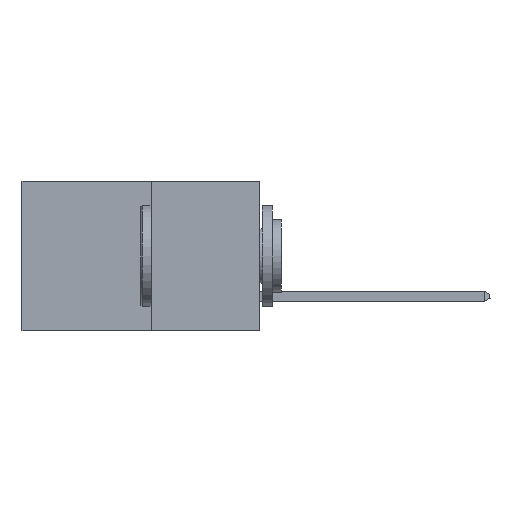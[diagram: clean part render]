
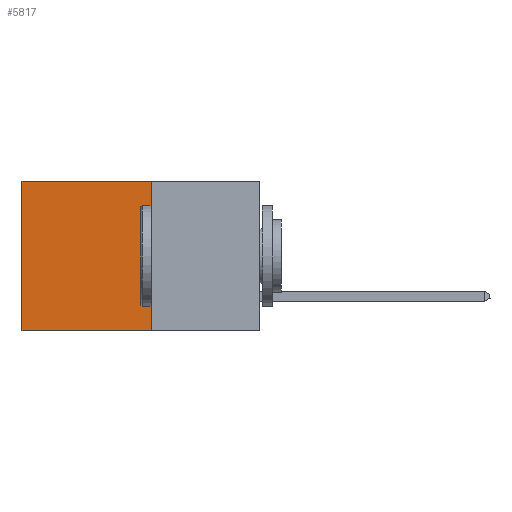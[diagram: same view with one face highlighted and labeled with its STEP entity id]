
A CAD part, left-side view. The second image highlights one B-rep face of the part: STEP entity #5817.
In plain terms, the highlighted planar face has unit normal (-1, 0, 0).
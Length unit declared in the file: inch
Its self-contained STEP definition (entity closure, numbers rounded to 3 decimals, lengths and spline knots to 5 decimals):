
#403 = EDGE_CURVE ( 'NONE', #16762, #11495, #9783, .T. ) ;
#775 = LINE ( 'NONE', #1571, #11149 ) ;
#1303 = FACE_OUTER_BOUND ( 'NONE', #5108, .T. ) ;
#1571 = CARTESIAN_POINT ( 'NONE',  ( 0.277, 0.27, -0.37 ) ) ;
#1641 = AXIS2_PLACEMENT_3D ( 'NONE', #7600, #4854, #14286 ) ;
#2205 = CARTESIAN_POINT ( 'NONE',  ( 0.277, 0.27, -0.37 ) ) ;
#3331 = CARTESIAN_POINT ( 'NONE',  ( 0.277, 0.27, 0. ) ) ;
#3481 = PLANE ( 'NONE',  #1641 ) ;
#4180 = ORIENTED_EDGE ( 'NONE', *, *, #403, .T. ) ;
#4215 = ORIENTED_EDGE ( 'NONE', *, *, #14540, .F. ) ;
#4248 = ORIENTED_EDGE ( 'NONE', *, *, #14178, .F. ) ;
#4289 = ORIENTED_EDGE ( 'NONE', *, *, #10012, .T. ) ;
#4854 = DIRECTION ( 'NONE',  ( 1., 0., 0. ) ) ;
#5108 = EDGE_LOOP ( 'NONE', ( #4180, #4215, #4248, #4289 ) ) ;
#5114 = CARTESIAN_POINT ( 'NONE',  ( 0.277, 0.59, 0. ) ) ;
#5817 = ADVANCED_FACE ( 'NONE', ( #1303 ), #3481, .F. ) ;
#6538 = CARTESIAN_POINT ( 'NONE',  ( 0.277, 0.27, -0.37 ) ) ;
#7092 = DIRECTION ( 'NONE',  ( 0., 1., 0. ) ) ;
#7600 = CARTESIAN_POINT ( 'NONE',  ( 0.277, 0.27, -0.37 ) ) ;
#7736 = DIRECTION ( 'NONE',  ( 0., 0., -1. ) ) ;
#9555 = LINE ( 'NONE', #2205, #16228 ) ;
#9783 = LINE ( 'NONE', #17522, #12895 ) ;
#10012 = EDGE_CURVE ( 'NONE', #14710, #16762, #16763, .T. ) ;
#11149 = VECTOR ( 'NONE', #7092, 39.37008 ) ;
#11495 = VERTEX_POINT ( 'NONE', #12813 ) ;
#12382 = VERTEX_POINT ( 'NONE', #6538 ) ;
#12776 = VECTOR ( 'NONE', #16448, 39.37008 ) ;
#12813 = CARTESIAN_POINT ( 'NONE',  ( 0.277, 0.59, -0.37 ) ) ;
#12895 = VECTOR ( 'NONE', #17347, 39.37008 ) ;
#14178 = EDGE_CURVE ( 'NONE', #14710, #12382, #9555, .T. ) ;
#14286 = DIRECTION ( 'NONE',  ( 0., 0., -1. ) ) ;
#14540 = EDGE_CURVE ( 'NONE', #12382, #11495, #775, .T. ) ;
#14710 = VERTEX_POINT ( 'NONE', #3331 ) ;
#16228 = VECTOR ( 'NONE', #7736, 39.37008 ) ;
#16448 = DIRECTION ( 'NONE',  ( 0., 1., 0. ) ) ;
#16509 = CARTESIAN_POINT ( 'NONE',  ( 0.277, 0.27, 0. ) ) ;
#16762 = VERTEX_POINT ( 'NONE', #5114 ) ;
#16763 = LINE ( 'NONE', #16509, #12776 ) ;
#17347 = DIRECTION ( 'NONE',  ( 0., 0., -1. ) ) ;
#17522 = CARTESIAN_POINT ( 'NONE',  ( 0.277, 0.59, -0.37 ) ) ;
